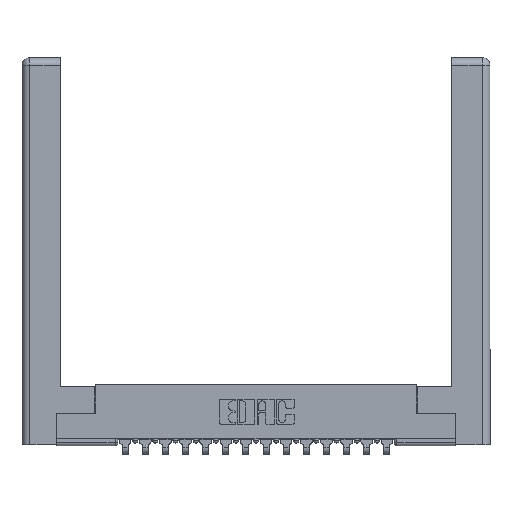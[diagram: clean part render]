
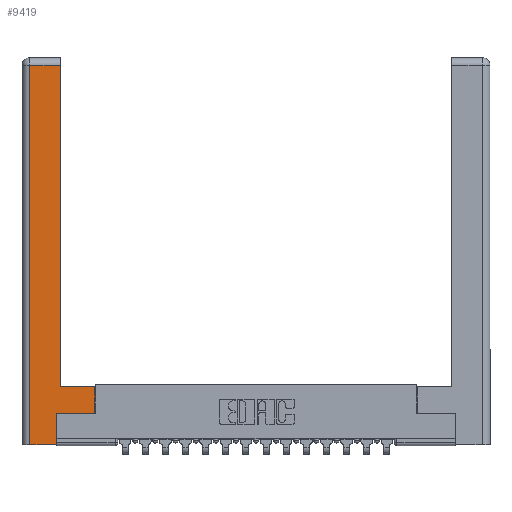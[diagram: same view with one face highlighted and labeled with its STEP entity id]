
A CAD part, top view. The second image highlights one B-rep face of the part: STEP entity #9419.
In plain terms, the highlighted planar face has unit normal (0, 0, 1).
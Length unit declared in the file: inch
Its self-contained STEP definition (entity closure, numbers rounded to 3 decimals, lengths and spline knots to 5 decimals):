
#91 = DIRECTION ( 'NONE',  ( 0., 1., 0. ) ) ;
#123 = FACE_OUTER_BOUND ( 'NONE', #7722, .T. ) ;
#204 = AXIS2_PLACEMENT_3D ( 'NONE', #1692, #3180, #4205 ) ;
#276 = VERTEX_POINT ( 'NONE', #17320 ) ;
#555 = ORIENTED_EDGE ( 'NONE', *, *, #10176, .T. ) ;
#1035 = VERTEX_POINT ( 'NONE', #13603 ) ;
#1169 = VECTOR ( 'NONE', #4833, 39.37008 ) ;
#1218 = CARTESIAN_POINT ( 'NONE',  ( 0.265, 0.245, 0. ) ) ;
#1574 = CARTESIAN_POINT ( 'NONE',  ( 0.295, 0.45, 0. ) ) ;
#1674 = VERTEX_POINT ( 'NONE', #13668 ) ;
#1692 = CARTESIAN_POINT ( 'NONE',  ( 0., 0., 0. ) ) ;
#1819 = LINE ( 'NONE', #7473, #17901 ) ;
#1850 = VECTOR ( 'NONE', #91, 39.37008 ) ;
#2010 = LINE ( 'NONE', #6190, #10897 ) ;
#2598 = LINE ( 'NONE', #11087, #1850 ) ;
#2987 = VECTOR ( 'NONE', #4699, 39.37008 ) ;
#3145 = EDGE_CURVE ( 'NONE', #6400, #3270, #8064, .T. ) ;
#3180 = DIRECTION ( 'NONE',  ( 0., 0., -1. ) ) ;
#3270 = VERTEX_POINT ( 'NONE', #10894 ) ;
#3726 = ORIENTED_EDGE ( 'NONE', *, *, #4626, .T. ) ;
#4205 = DIRECTION ( 'NONE',  ( -1., 0., 0. ) ) ;
#4371 = PLANE ( 'NONE',  #204 ) ;
#4626 = EDGE_CURVE ( 'NONE', #8088, #6400, #13657, .T. ) ;
#4699 = DIRECTION ( 'NONE',  ( -1., 0., 0. ) ) ;
#4833 = DIRECTION ( 'NONE',  ( 0., -1., 0. ) ) ;
#5178 = LINE ( 'NONE', #16396, #16708 ) ;
#5676 = VECTOR ( 'NONE', #9785, 39.37008 ) ;
#6047 = ORIENTED_EDGE ( 'NONE', *, *, #3145, .T. ) ;
#6190 = CARTESIAN_POINT ( 'NONE',  ( 0.565, 0.45, 0. ) ) ;
#6400 = VERTEX_POINT ( 'NONE', #13811 ) ;
#6643 = ORIENTED_EDGE ( 'NONE', *, *, #15035, .T. ) ;
#7017 = CARTESIAN_POINT ( 'NONE',  ( 0.265, 0., 0. ) ) ;
#7473 = CARTESIAN_POINT ( 'NONE',  ( 0.565, 0.245, 0. ) ) ;
#7686 = VERTEX_POINT ( 'NONE', #17972 ) ;
#7722 = EDGE_LOOP ( 'NONE', ( #555, #14158, #3726, #6047, #15135, #18000, #11973, #6643 ) ) ;
#8064 = LINE ( 'NONE', #7017, #5676 ) ;
#8088 = VERTEX_POINT ( 'NONE', #16388 ) ;
#9419 = ADVANCED_FACE ( 'NONE', ( #123 ), #4371, .F. ) ;
#9629 = EDGE_CURVE ( 'NONE', #3270, #7686, #15222, .T. ) ;
#9785 = DIRECTION ( 'NONE',  ( 1., 0., 0. ) ) ;
#10158 = LINE ( 'NONE', #1574, #2987 ) ;
#10159 = EDGE_CURVE ( 'NONE', #1035, #8088, #5178, .T. ) ;
#10176 = EDGE_CURVE ( 'NONE', #17584, #1035, #2598, .T. ) ;
#10752 = CARTESIAN_POINT ( 'NONE',  ( 0.295, 0.45, 0. ) ) ;
#10894 = CARTESIAN_POINT ( 'NONE',  ( 0.265, 0., 0. ) ) ;
#10897 = VECTOR ( 'NONE', #16200, 39.37008 ) ;
#11087 = CARTESIAN_POINT ( 'NONE',  ( 0.295, 3., 0. ) ) ;
#11137 = VECTOR ( 'NONE', #16516, 39.37008 ) ;
#11973 = ORIENTED_EDGE ( 'NONE', *, *, #13315, .T. ) ;
#12013 = CARTESIAN_POINT ( 'NONE',  ( 0.0615, 0., 0. ) ) ;
#12186 = EDGE_CURVE ( 'NONE', #7686, #1674, #1819, .T. ) ;
#12369 = DIRECTION ( 'NONE',  ( -1., 0., 0. ) ) ;
#13067 = DIRECTION ( 'NONE',  ( 1., 0., 0. ) ) ;
#13315 = EDGE_CURVE ( 'NONE', #1674, #276, #2010, .T. ) ;
#13603 = CARTESIAN_POINT ( 'NONE',  ( 0.295, 2.94, 0. ) ) ;
#13657 = LINE ( 'NONE', #12013, #1169 ) ;
#13668 = CARTESIAN_POINT ( 'NONE',  ( 0.565, 0.245, 0. ) ) ;
#13811 = CARTESIAN_POINT ( 'NONE',  ( 0.0615, 0., 0. ) ) ;
#14158 = ORIENTED_EDGE ( 'NONE', *, *, #10159, .T. ) ;
#15035 = EDGE_CURVE ( 'NONE', #276, #17584, #10158, .T. ) ;
#15135 = ORIENTED_EDGE ( 'NONE', *, *, #9629, .T. ) ;
#15222 = LINE ( 'NONE', #1218, #11137 ) ;
#16200 = DIRECTION ( 'NONE',  ( 0., 1., 0. ) ) ;
#16388 = CARTESIAN_POINT ( 'NONE',  ( 0.0615, 2.94, 0. ) ) ;
#16396 = CARTESIAN_POINT ( 'NONE',  ( 0.0615, 2.94, 0. ) ) ;
#16516 = DIRECTION ( 'NONE',  ( 0., 1., 0. ) ) ;
#16708 = VECTOR ( 'NONE', #12369, 39.37008 ) ;
#17320 = CARTESIAN_POINT ( 'NONE',  ( 0.565, 0.45, 0. ) ) ;
#17584 = VERTEX_POINT ( 'NONE', #10752 ) ;
#17901 = VECTOR ( 'NONE', #13067, 39.37008 ) ;
#17972 = CARTESIAN_POINT ( 'NONE',  ( 0.265, 0.245, 0. ) ) ;
#18000 = ORIENTED_EDGE ( 'NONE', *, *, #12186, .T. ) ;
